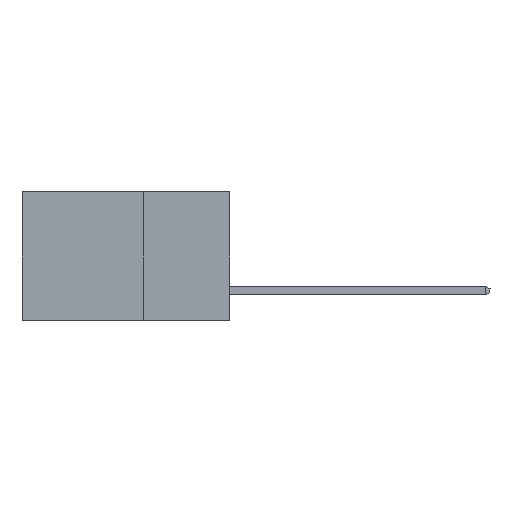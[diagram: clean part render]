
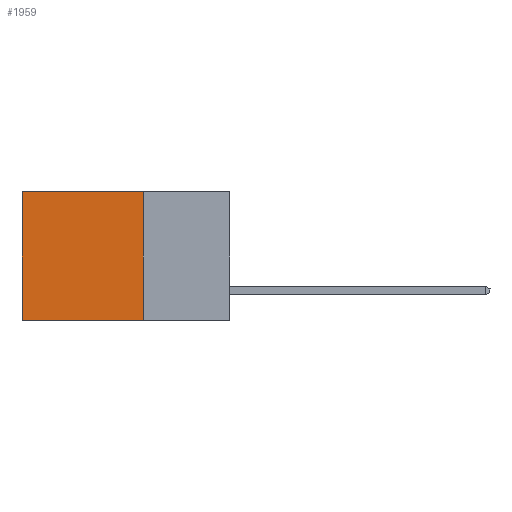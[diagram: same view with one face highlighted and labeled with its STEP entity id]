
A CAD part, left-side view. The second image highlights one B-rep face of the part: STEP entity #1959.
In plain terms, the highlighted planar face has unit normal (-1, 0, 0).
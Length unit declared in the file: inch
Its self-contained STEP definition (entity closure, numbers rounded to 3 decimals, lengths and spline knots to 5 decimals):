
#49 = EDGE_CURVE ( 'NONE', #4571, #10410, #13170, .T. ) ;
#530 = ORIENTED_EDGE ( 'NONE', *, *, #49, .F. ) ;
#1618 = EDGE_CURVE ( 'NONE', #4783, #12567, #5579, .T. ) ;
#1959 = ADVANCED_FACE ( 'NONE', ( #2507 ), #9236, .F. ) ;
#2175 = AXIS2_PLACEMENT_3D ( 'NONE', #15597, #11497, #4313 ) ;
#2195 = ORIENTED_EDGE ( 'NONE', *, *, #1618, .T. ) ;
#2319 = ORIENTED_EDGE ( 'NONE', *, *, #5151, .T. ) ;
#2507 = FACE_OUTER_BOUND ( 'NONE', #7908, .T. ) ;
#3547 = CARTESIAN_POINT ( 'NONE',  ( 0.2615, 0.25, -0.37 ) ) ;
#3899 = DIRECTION ( 'NONE',  ( 0., 1., 0. ) ) ;
#4313 = DIRECTION ( 'NONE',  ( 0., 0., -1. ) ) ;
#4571 = VERTEX_POINT ( 'NONE', #15376 ) ;
#4596 = CARTESIAN_POINT ( 'NONE',  ( 0.2615, 0.6, -0.37 ) ) ;
#4693 = VECTOR ( 'NONE', #15738, 39.37008 ) ;
#4705 = DIRECTION ( 'NONE',  ( 0., 1., 0. ) ) ;
#4783 = VERTEX_POINT ( 'NONE', #7942 ) ;
#5151 = EDGE_CURVE ( 'NONE', #4571, #4783, #10158, .T. ) ;
#5579 = LINE ( 'NONE', #4596, #14433 ) ;
#5941 = LINE ( 'NONE', #15986, #15132 ) ;
#6531 = ORIENTED_EDGE ( 'NONE', *, *, #14239, .F. ) ;
#7282 = CARTESIAN_POINT ( 'NONE',  ( 0.2615, 0.25, -0.37 ) ) ;
#7908 = EDGE_LOOP ( 'NONE', ( #2195, #6531, #530, #2319 ) ) ;
#7942 = CARTESIAN_POINT ( 'NONE',  ( 0.2615, 0.6, 0. ) ) ;
#9236 = PLANE ( 'NONE',  #2175 ) ;
#10158 = LINE ( 'NONE', #15192, #11037 ) ;
#10410 = VERTEX_POINT ( 'NONE', #3547 ) ;
#10604 = DIRECTION ( 'NONE',  ( 0., 0., -1. ) ) ;
#11037 = VECTOR ( 'NONE', #3899, 39.37008 ) ;
#11497 = DIRECTION ( 'NONE',  ( 1., 0., 0. ) ) ;
#12567 = VERTEX_POINT ( 'NONE', #16151 ) ;
#13170 = LINE ( 'NONE', #7282, #4693 ) ;
#14239 = EDGE_CURVE ( 'NONE', #10410, #12567, #5941, .T. ) ;
#14433 = VECTOR ( 'NONE', #10604, 39.37008 ) ;
#15132 = VECTOR ( 'NONE', #4705, 39.37008 ) ;
#15192 = CARTESIAN_POINT ( 'NONE',  ( 0.2615, 0.25, 0. ) ) ;
#15376 = CARTESIAN_POINT ( 'NONE',  ( 0.2615, 0.25, 0. ) ) ;
#15597 = CARTESIAN_POINT ( 'NONE',  ( 0.2615, 0.25, -0.37 ) ) ;
#15738 = DIRECTION ( 'NONE',  ( 0., 0., -1. ) ) ;
#15986 = CARTESIAN_POINT ( 'NONE',  ( 0.2615, 0.25, -0.37 ) ) ;
#16151 = CARTESIAN_POINT ( 'NONE',  ( 0.2615, 0.6, -0.37 ) ) ;
